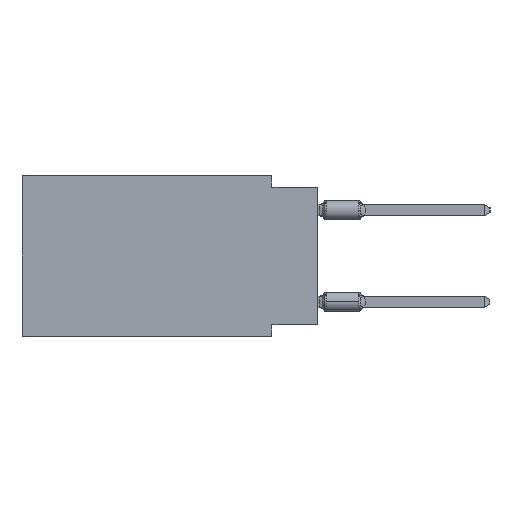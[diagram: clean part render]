
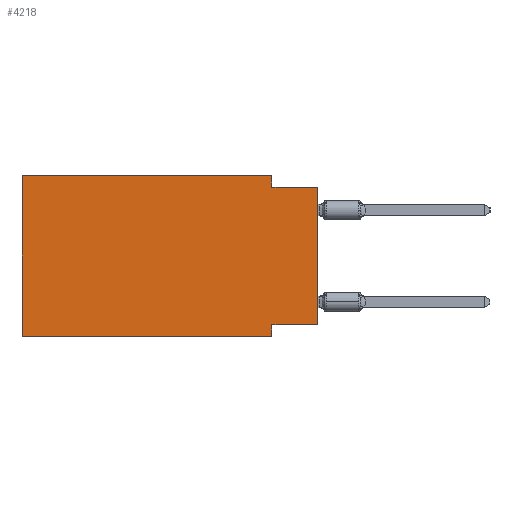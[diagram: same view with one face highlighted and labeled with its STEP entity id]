
A CAD part, left-side view. The second image highlights one B-rep face of the part: STEP entity #4218.
In plain terms, the highlighted planar face has unit normal (-1, 0, 0).
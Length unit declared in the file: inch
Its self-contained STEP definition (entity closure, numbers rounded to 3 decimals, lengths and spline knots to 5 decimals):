
#57 = VECTOR ( 'NONE', #17472, 39.37008 ) ;
#3024 = LINE ( 'NONE', #16708, #10259 ) ;
#3169 = CARTESIAN_POINT ( 'NONE',  ( 0., 0.645, 0. ) ) ;
#3195 = VERTEX_POINT ( 'NONE', #21835 ) ;
#3407 = EDGE_CURVE ( 'NONE', #8738, #21468, #19355, .T. ) ;
#3609 = DIRECTION ( 'NONE',  ( 1., 0., 0. ) ) ;
#4218 = ADVANCED_FACE ( 'NONE', ( #30826 ), #17112, .F. ) ;
#5289 = DIRECTION ( 'NONE',  ( 0., 0., -1. ) ) ;
#5868 = CARTESIAN_POINT ( 'NONE',  ( 0., 0., -0.025 ) ) ;
#6610 = CARTESIAN_POINT ( 'NONE',  ( 0., 0., -0.325 ) ) ;
#6647 = LINE ( 'NONE', #28684, #57 ) ;
#7069 = ORIENTED_EDGE ( 'NONE', *, *, #3407, .F. ) ;
#7114 = EDGE_CURVE ( 'NONE', #8357, #12732, #12630, .T. ) ;
#7440 = EDGE_CURVE ( 'NONE', #18350, #3195, #14349, .T. ) ;
#8357 = VERTEX_POINT ( 'NONE', #6610 ) ;
#8725 = CARTESIAN_POINT ( 'NONE',  ( 0., 0.645, 0. ) ) ;
#8738 = VERTEX_POINT ( 'NONE', #8725 ) ;
#9232 = CARTESIAN_POINT ( 'NONE',  ( 0., 0.1, 0. ) ) ;
#9580 = DIRECTION ( 'NONE',  ( 0., 0., -1. ) ) ;
#10259 = VECTOR ( 'NONE', #16540, 39.37008 ) ;
#10677 = CARTESIAN_POINT ( 'NONE',  ( 0., 0.1, -0.325 ) ) ;
#11707 = LINE ( 'NONE', #9232, #18786 ) ;
#12630 = LINE ( 'NONE', #19912, #13601 ) ;
#12732 = VERTEX_POINT ( 'NONE', #10677 ) ;
#12828 = CARTESIAN_POINT ( 'NONE',  ( 0., 0.645, -0.35 ) ) ;
#13052 = DIRECTION ( 'NONE',  ( 0., 0., 1. ) ) ;
#13230 = LINE ( 'NONE', #24057, #23325 ) ;
#13601 = VECTOR ( 'NONE', #30771, 39.37008 ) ;
#13990 = CARTESIAN_POINT ( 'NONE',  ( 0., 0.645, -0.35 ) ) ;
#14009 = DIRECTION ( 'NONE',  ( 0., -1., 0. ) ) ;
#14349 = LINE ( 'NONE', #13990, #34085 ) ;
#14445 = DIRECTION ( 'NONE',  ( 0., 0., -1. ) ) ;
#15369 = ORIENTED_EDGE ( 'NONE', *, *, #24020, .F. ) ;
#16540 = DIRECTION ( 'NONE',  ( 0., 0., 1. ) ) ;
#16708 = CARTESIAN_POINT ( 'NONE',  ( 0., 0.645, 0. ) ) ;
#16748 = CARTESIAN_POINT ( 'NONE',  ( 0., 0.1, -0.025 ) ) ;
#17112 = PLANE ( 'NONE',  #25522 ) ;
#17356 = ORIENTED_EDGE ( 'NONE', *, *, #22614, .T. ) ;
#17472 = DIRECTION ( 'NONE',  ( 0., -1., 0. ) ) ;
#18350 = VERTEX_POINT ( 'NONE', #12828 ) ;
#18721 = CARTESIAN_POINT ( 'NONE',  ( 0., 0.1, 0. ) ) ;
#18786 = VECTOR ( 'NONE', #9580, 39.37008 ) ;
#18869 = EDGE_CURVE ( 'NONE', #12732, #3195, #24125, .T. ) ;
#19355 = LINE ( 'NONE', #3169, #32960 ) ;
#19912 = CARTESIAN_POINT ( 'NONE',  ( 0., 0., -0.325 ) ) ;
#20347 = ORIENTED_EDGE ( 'NONE', *, *, #33312, .F. ) ;
#21468 = VERTEX_POINT ( 'NONE', #18721 ) ;
#21627 = ORIENTED_EDGE ( 'NONE', *, *, #7440, .T. ) ;
#21835 = CARTESIAN_POINT ( 'NONE',  ( 0., 0.1, -0.35 ) ) ;
#22614 = EDGE_CURVE ( 'NONE', #8357, #29288, #13230, .T. ) ;
#23325 = VECTOR ( 'NONE', #13052, 39.37008 ) ;
#24020 = EDGE_CURVE ( 'NONE', #30081, #29288, #6647, .T. ) ;
#24057 = CARTESIAN_POINT ( 'NONE',  ( 0., 0., 0. ) ) ;
#24125 = LINE ( 'NONE', #34989, #32181 ) ;
#25522 = AXIS2_PLACEMENT_3D ( 'NONE', #27971, #3609, #14445 ) ;
#27971 = CARTESIAN_POINT ( 'NONE',  ( 0., 0.645, 0. ) ) ;
#28353 = EDGE_LOOP ( 'NONE', ( #17356, #15369, #20347, #7069, #34672, #21627, #34990, #29026 ) ) ;
#28684 = CARTESIAN_POINT ( 'NONE',  ( 0., 0., -0.025 ) ) ;
#29026 = ORIENTED_EDGE ( 'NONE', *, *, #7114, .F. ) ;
#29288 = VERTEX_POINT ( 'NONE', #5868 ) ;
#30081 = VERTEX_POINT ( 'NONE', #16748 ) ;
#30771 = DIRECTION ( 'NONE',  ( 0., 1., 0. ) ) ;
#30826 = FACE_OUTER_BOUND ( 'NONE', #28353, .T. ) ;
#32181 = VECTOR ( 'NONE', #5289, 39.37008 ) ;
#32801 = EDGE_CURVE ( 'NONE', #18350, #8738, #3024, .T. ) ;
#32856 = DIRECTION ( 'NONE',  ( 0., -1., 0. ) ) ;
#32960 = VECTOR ( 'NONE', #14009, 39.37008 ) ;
#33312 = EDGE_CURVE ( 'NONE', #21468, #30081, #11707, .T. ) ;
#34085 = VECTOR ( 'NONE', #32856, 39.37008 ) ;
#34672 = ORIENTED_EDGE ( 'NONE', *, *, #32801, .F. ) ;
#34989 = CARTESIAN_POINT ( 'NONE',  ( 0., 0.1, -0.35 ) ) ;
#34990 = ORIENTED_EDGE ( 'NONE', *, *, #18869, .F. ) ;
